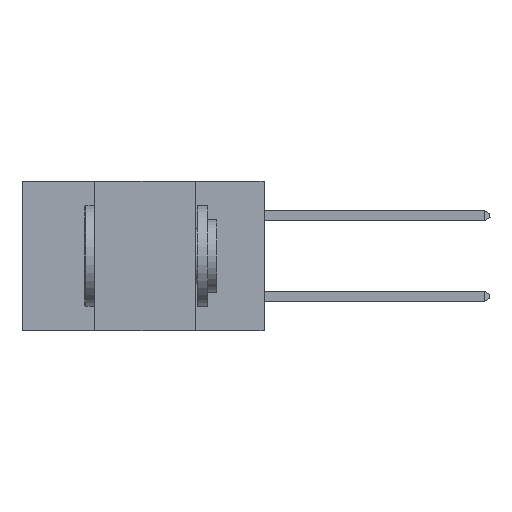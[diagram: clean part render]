
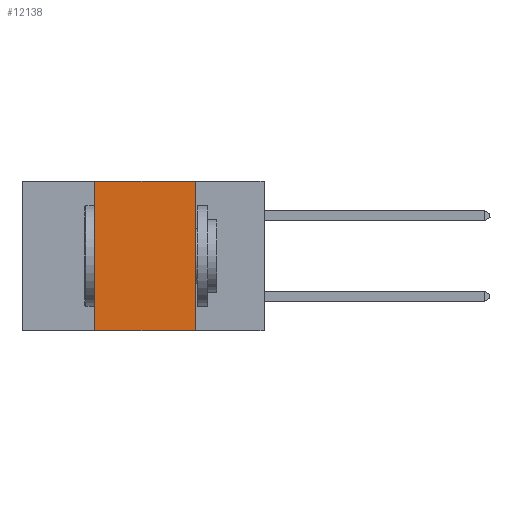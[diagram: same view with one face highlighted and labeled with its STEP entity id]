
A CAD part, left-side view. The second image highlights one B-rep face of the part: STEP entity #12138.
In plain terms, the highlighted planar face has unit normal (-1, 0, 0).
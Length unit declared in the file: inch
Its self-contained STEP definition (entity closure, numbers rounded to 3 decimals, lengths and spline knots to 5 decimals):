
#413 = LINE ( 'NONE', #12277, #4304 ) ;
#441 = DIRECTION ( 'NONE',  ( 0., -1., 0. ) ) ;
#452 = CARTESIAN_POINT ( 'NONE',  ( 0., 0.6, 0. ) ) ;
#677 = LINE ( 'NONE', #4566, #10990 ) ;
#734 = VERTEX_POINT ( 'NONE', #8293 ) ;
#1408 = PLANE ( 'NONE',  #13334 ) ;
#2498 = ORIENTED_EDGE ( 'NONE', *, *, #12213, .F. ) ;
#2624 = ORIENTED_EDGE ( 'NONE', *, *, #8408, .F. ) ;
#3229 = FACE_OUTER_BOUND ( 'NONE', #6968, .T. ) ;
#4180 = CARTESIAN_POINT ( 'NONE',  ( 0., 0.42, 0. ) ) ;
#4304 = VECTOR ( 'NONE', #12416, 39.37008 ) ;
#4342 = VECTOR ( 'NONE', #13005, 39.37008 ) ;
#4566 = CARTESIAN_POINT ( 'NONE',  ( 0., 0.6, -0.37 ) ) ;
#4571 = CARTESIAN_POINT ( 'NONE',  ( 0., 0.42, 0. ) ) ;
#4851 = ORIENTED_EDGE ( 'NONE', *, *, #12781, .T. ) ;
#5119 = VERTEX_POINT ( 'NONE', #14007 ) ;
#5446 = ORIENTED_EDGE ( 'NONE', *, *, #7806, .F. ) ;
#5518 = LINE ( 'NONE', #4180, #4342 ) ;
#5965 = LINE ( 'NONE', #11309, #12353 ) ;
#6695 = DIRECTION ( 'NONE',  ( 0., 0., -1. ) ) ;
#6968 = EDGE_LOOP ( 'NONE', ( #2624, #2498, #5446, #4851 ) ) ;
#7806 = EDGE_CURVE ( 'NONE', #5119, #12446, #5518, .T. ) ;
#7834 = VERTEX_POINT ( 'NONE', #8920 ) ;
#8293 = CARTESIAN_POINT ( 'NONE',  ( 0., 0.17, 0. ) ) ;
#8408 = EDGE_CURVE ( 'NONE', #734, #7834, #413, .T. ) ;
#8920 = CARTESIAN_POINT ( 'NONE',  ( 0., 0.17, -0.37 ) ) ;
#10990 = VECTOR ( 'NONE', #441, 39.37008 ) ;
#11309 = CARTESIAN_POINT ( 'NONE',  ( 0., 0.6, 0. ) ) ;
#12138 = ADVANCED_FACE ( 'NONE', ( #3229 ), #1408, .F. ) ;
#12197 = DIRECTION ( 'NONE',  ( 0., -1., 0. ) ) ;
#12213 = EDGE_CURVE ( 'NONE', #12446, #734, #5965, .T. ) ;
#12277 = CARTESIAN_POINT ( 'NONE',  ( 0., 0.17, 0. ) ) ;
#12353 = VECTOR ( 'NONE', #12197, 39.37008 ) ;
#12416 = DIRECTION ( 'NONE',  ( 0., 0., -1. ) ) ;
#12446 = VERTEX_POINT ( 'NONE', #4571 ) ;
#12781 = EDGE_CURVE ( 'NONE', #5119, #7834, #677, .T. ) ;
#13005 = DIRECTION ( 'NONE',  ( 0., 0., 1. ) ) ;
#13334 = AXIS2_PLACEMENT_3D ( 'NONE', #452, #13347, #6695 ) ;
#13347 = DIRECTION ( 'NONE',  ( 1., 0., 0. ) ) ;
#14007 = CARTESIAN_POINT ( 'NONE',  ( 0., 0.42, -0.37 ) ) ;
